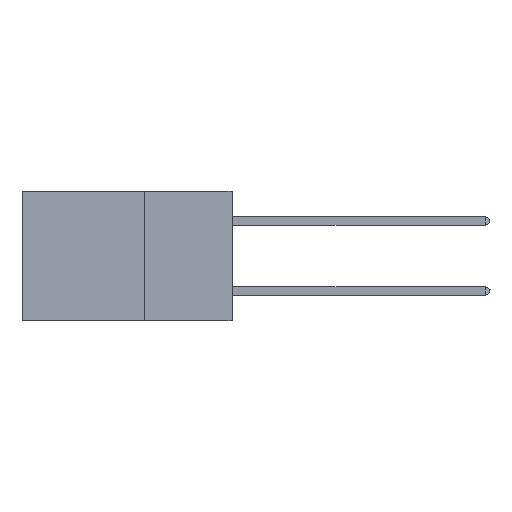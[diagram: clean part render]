
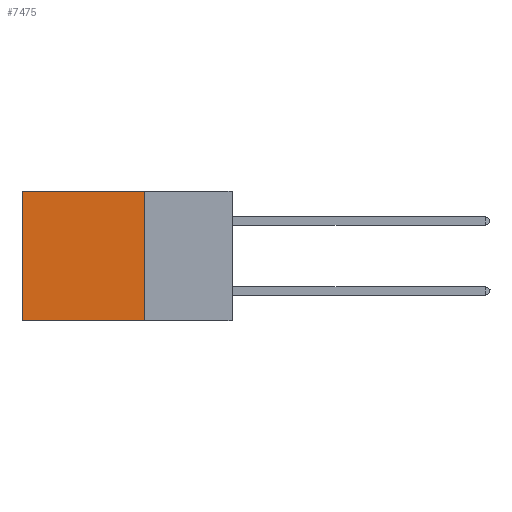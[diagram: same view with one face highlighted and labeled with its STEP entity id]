
A CAD part, left-side view. The second image highlights one B-rep face of the part: STEP entity #7475.
In plain terms, the highlighted planar face has unit normal (-1, 0, 0).
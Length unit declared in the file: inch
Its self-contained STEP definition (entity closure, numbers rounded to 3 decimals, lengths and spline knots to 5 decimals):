
#254 = CARTESIAN_POINT ( 'NONE',  ( 0.2875, 0.25, 0. ) ) ;
#611 = LINE ( 'NONE', #16312, #8918 ) ;
#2215 = CARTESIAN_POINT ( 'NONE',  ( 0.2875, 0.6, 0. ) ) ;
#2318 = LINE ( 'NONE', #10184, #18139 ) ;
#2673 = VERTEX_POINT ( 'NONE', #20298 ) ;
#6296 = AXIS2_PLACEMENT_3D ( 'NONE', #15153, #21206, #13220 ) ;
#6836 = VERTEX_POINT ( 'NONE', #2215 ) ;
#7286 = PLANE ( 'NONE',  #6296 ) ;
#7475 = ADVANCED_FACE ( 'NONE', ( #24922 ), #7286, .F. ) ;
#7582 = CARTESIAN_POINT ( 'NONE',  ( 0.2875, 0.25, -0.37 ) ) ;
#8087 = CARTESIAN_POINT ( 'NONE',  ( 0.2875, 0.25, -0.37 ) ) ;
#8255 = DIRECTION ( 'NONE',  ( 0., 1., 0. ) ) ;
#8866 = VECTOR ( 'NONE', #13069, 39.37008 ) ;
#8918 = VECTOR ( 'NONE', #14886, 39.37008 ) ;
#9337 = CARTESIAN_POINT ( 'NONE',  ( 0.2875, 0.6, 0. ) ) ;
#10184 = CARTESIAN_POINT ( 'NONE',  ( 0.2875, 0.25, 0. ) ) ;
#11490 = EDGE_CURVE ( 'NONE', #23330, #23356, #611, .T. ) ;
#12808 = ORIENTED_EDGE ( 'NONE', *, *, #19594, .F. ) ;
#13069 = DIRECTION ( 'NONE',  ( 0., 0., -1. ) ) ;
#13134 = DIRECTION ( 'NONE',  ( 0., 1., 0. ) ) ;
#13220 = DIRECTION ( 'NONE',  ( 0., 0., -1. ) ) ;
#13710 = ORIENTED_EDGE ( 'NONE', *, *, #17975, .T. ) ;
#14454 = ORIENTED_EDGE ( 'NONE', *, *, #11490, .F. ) ;
#14886 = DIRECTION ( 'NONE',  ( 0., 0., -1. ) ) ;
#15153 = CARTESIAN_POINT ( 'NONE',  ( 0.2875, 0.25, 0. ) ) ;
#15633 = LINE ( 'NONE', #9337, #8866 ) ;
#16272 = VECTOR ( 'NONE', #13134, 39.37008 ) ;
#16312 = CARTESIAN_POINT ( 'NONE',  ( 0.2875, 0.25, 0. ) ) ;
#16870 = LINE ( 'NONE', #7582, #16272 ) ;
#17975 = EDGE_CURVE ( 'NONE', #23330, #6836, #2318, .T. ) ;
#18139 = VECTOR ( 'NONE', #8255, 39.37008 ) ;
#18691 = EDGE_CURVE ( 'NONE', #6836, #2673, #15633, .T. ) ;
#19036 = EDGE_LOOP ( 'NONE', ( #23901, #12808, #14454, #13710 ) ) ;
#19594 = EDGE_CURVE ( 'NONE', #23356, #2673, #16870, .T. ) ;
#20298 = CARTESIAN_POINT ( 'NONE',  ( 0.2875, 0.6, -0.37 ) ) ;
#21206 = DIRECTION ( 'NONE',  ( 1., 0., 0. ) ) ;
#23330 = VERTEX_POINT ( 'NONE', #254 ) ;
#23356 = VERTEX_POINT ( 'NONE', #8087 ) ;
#23901 = ORIENTED_EDGE ( 'NONE', *, *, #18691, .T. ) ;
#24922 = FACE_OUTER_BOUND ( 'NONE', #19036, .T. ) ;
